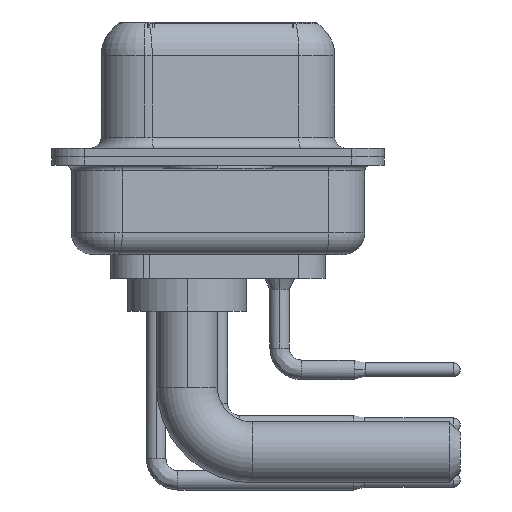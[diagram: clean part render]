
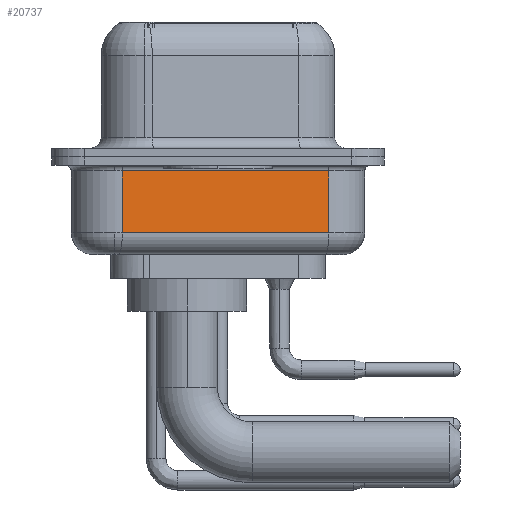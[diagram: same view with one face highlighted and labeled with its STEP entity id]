
A CAD part, left-side view. The second image highlights one B-rep face of the part: STEP entity #20737.
In plain terms, the highlighted planar face has unit normal (-0.985, -0.174, 0).
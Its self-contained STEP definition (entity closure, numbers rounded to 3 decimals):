
#1735 = DIRECTION ( 'NONE',  ( 0., 0., 1. ) ) ;
#3169 = EDGE_LOOP ( 'NONE', ( #12912, #16834, #27175, #25977 ) ) ;
#3680 = LINE ( 'NONE', #3938, #7254 ) ;
#3938 = CARTESIAN_POINT ( 'NONE',  ( 2.93, 4.403, -0.65 ) ) ;
#4588 = DIRECTION ( 'NONE',  ( -0.174, 0.985, 0. ) ) ;
#5019 = CARTESIAN_POINT ( 'NONE',  ( 2.93, 4.403, -4.5 ) ) ;
#5919 = CARTESIAN_POINT ( 'NONE',  ( 2.93, 4.403, -3.5 ) ) ;
#7152 = VERTEX_POINT ( 'NONE', #5919 ) ;
#7254 = VECTOR ( 'NONE', #25028, 1000. ) ;
#8129 = CARTESIAN_POINT ( 'NONE',  ( 2.93, 4.403, -4.5 ) ) ;
#10179 = VECTOR ( 'NONE', #1735, 1000. ) ;
#10226 = DIRECTION ( 'NONE',  ( 0., 0., 1. ) ) ;
#10880 = VERTEX_POINT ( 'NONE', #18805 ) ;
#11001 = PLANE ( 'NONE',  #15508 ) ;
#11638 = VERTEX_POINT ( 'NONE', #27129 ) ;
#12337 = LINE ( 'NONE', #20844, #10179 ) ;
#12912 = ORIENTED_EDGE ( 'NONE', *, *, #25955, .F. ) ;
#13508 = EDGE_CURVE ( 'NONE', #7152, #10880, #25165, .T. ) ;
#14867 = VECTOR ( 'NONE', #10226, 1000. ) ;
#15508 = AXIS2_PLACEMENT_3D ( 'NONE', #5019, #19923, #4588 ) ;
#16834 = ORIENTED_EDGE ( 'NONE', *, *, #13508, .T. ) ;
#18805 = CARTESIAN_POINT ( 'NONE',  ( 4.605, -5.097, -3.5 ) ) ;
#18983 = EDGE_CURVE ( 'NONE', #10880, #11638, #12337, .T. ) ;
#19923 = DIRECTION ( 'NONE',  ( 0.985, 0.174, 0. ) ) ;
#20737 = ADVANCED_FACE ( 'NONE', ( #21600 ), #11001, .F. ) ;
#20844 = CARTESIAN_POINT ( 'NONE',  ( 4.605, -5.097, -4.5 ) ) ;
#21099 = DIRECTION ( 'NONE',  ( 0.174, -0.985, 0. ) ) ;
#21236 = CARTESIAN_POINT ( 'NONE',  ( 2.93, 4.403, -3.5 ) ) ;
#21600 = FACE_OUTER_BOUND ( 'NONE', #3169, .T. ) ;
#21981 = VECTOR ( 'NONE', #21099, 1000. ) ;
#24321 = CARTESIAN_POINT ( 'NONE',  ( 2.93, 4.403, -0.65 ) ) ;
#24506 = VERTEX_POINT ( 'NONE', #24321 ) ;
#24886 = LINE ( 'NONE', #8129, #14867 ) ;
#25028 = DIRECTION ( 'NONE',  ( -0.174, 0.985, 0. ) ) ;
#25165 = LINE ( 'NONE', #21236, #21981 ) ;
#25955 = EDGE_CURVE ( 'NONE', #7152, #24506, #24886, .T. ) ;
#25977 = ORIENTED_EDGE ( 'NONE', *, *, #25996, .T. ) ;
#25996 = EDGE_CURVE ( 'NONE', #11638, #24506, #3680, .T. ) ;
#27129 = CARTESIAN_POINT ( 'NONE',  ( 4.605, -5.097, -0.65 ) ) ;
#27175 = ORIENTED_EDGE ( 'NONE', *, *, #18983, .T. ) ;
